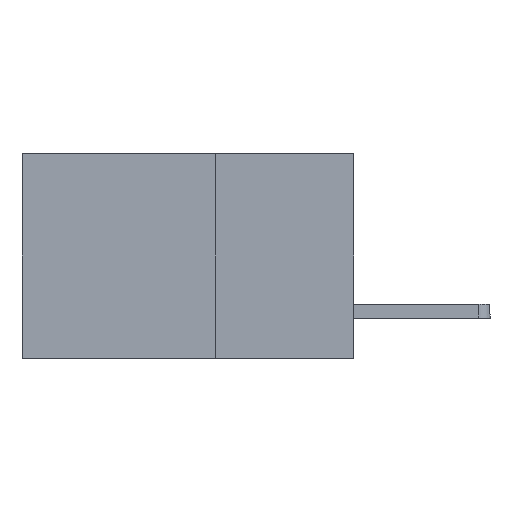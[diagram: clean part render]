
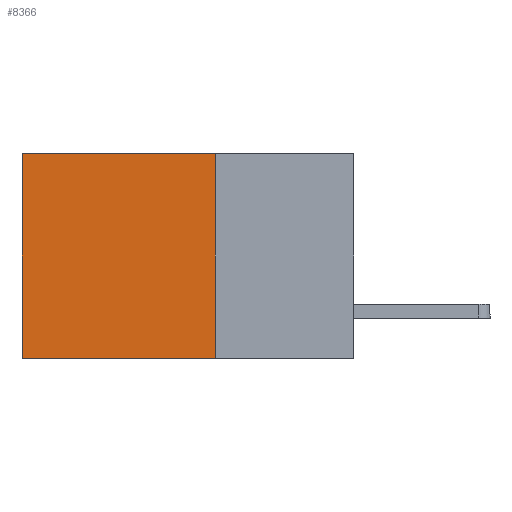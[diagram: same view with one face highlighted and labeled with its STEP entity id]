
A CAD part, left-side view. The second image highlights one B-rep face of the part: STEP entity #8366.
In plain terms, the highlighted planar face has unit normal (-1, 0, 0).
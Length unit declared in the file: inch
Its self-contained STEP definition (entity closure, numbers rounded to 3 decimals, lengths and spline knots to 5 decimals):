
#28 = LINE ( 'NONE', #761, #9189 ) ;
#244 = VECTOR ( 'NONE', #1741, 39.37008 ) ;
#370 = DIRECTION ( 'NONE',  ( 0., 1., 0. ) ) ;
#462 = ORIENTED_EDGE ( 'NONE', *, *, #7740, .T. ) ;
#761 = CARTESIAN_POINT ( 'NONE',  ( 0.2875, 0.6, 0. ) ) ;
#771 = CARTESIAN_POINT ( 'NONE',  ( 0.2875, 0.25, -0.37 ) ) ;
#1051 = VERTEX_POINT ( 'NONE', #2769 ) ;
#1451 = EDGE_LOOP ( 'NONE', ( #462, #9881, #8001, #5736 ) ) ;
#1741 = DIRECTION ( 'NONE',  ( 0., 1., 0. ) ) ;
#1756 = DIRECTION ( 'NONE',  ( 1., 0., 0. ) ) ;
#1991 = LINE ( 'NONE', #7699, #8394 ) ;
#2594 = EDGE_CURVE ( 'NONE', #10038, #2870, #1991, .T. ) ;
#2769 = CARTESIAN_POINT ( 'NONE',  ( 0.2875, 0.6, -0.37 ) ) ;
#2828 = LINE ( 'NONE', #771, #244 ) ;
#2870 = VERTEX_POINT ( 'NONE', #9667 ) ;
#4495 = PLANE ( 'NONE',  #5486 ) ;
#4669 = VERTEX_POINT ( 'NONE', #6980 ) ;
#4952 = EDGE_CURVE ( 'NONE', #2870, #1051, #2828, .T. ) ;
#4968 = LINE ( 'NONE', #9167, #5514 ) ;
#5260 = FACE_OUTER_BOUND ( 'NONE', #1451, .T. ) ;
#5486 = AXIS2_PLACEMENT_3D ( 'NONE', #7082, #1756, #7900 ) ;
#5514 = VECTOR ( 'NONE', #370, 39.37008 ) ;
#5736 = ORIENTED_EDGE ( 'NONE', *, *, #8901, .T. ) ;
#6980 = CARTESIAN_POINT ( 'NONE',  ( 0.2875, 0.6, 0. ) ) ;
#7082 = CARTESIAN_POINT ( 'NONE',  ( 0.2875, 0.25, 0. ) ) ;
#7569 = DIRECTION ( 'NONE',  ( 0., 0., -1. ) ) ;
#7699 = CARTESIAN_POINT ( 'NONE',  ( 0.2875, 0.25, 0. ) ) ;
#7740 = EDGE_CURVE ( 'NONE', #4669, #1051, #28, .T. ) ;
#7900 = DIRECTION ( 'NONE',  ( 0., 0., -1. ) ) ;
#8001 = ORIENTED_EDGE ( 'NONE', *, *, #2594, .F. ) ;
#8366 = ADVANCED_FACE ( 'NONE', ( #5260 ), #4495, .F. ) ;
#8394 = VECTOR ( 'NONE', #7569, 39.37008 ) ;
#8901 = EDGE_CURVE ( 'NONE', #10038, #4669, #4968, .T. ) ;
#9167 = CARTESIAN_POINT ( 'NONE',  ( 0.2875, 0.25, 0. ) ) ;
#9189 = VECTOR ( 'NONE', #11030, 39.37008 ) ;
#9667 = CARTESIAN_POINT ( 'NONE',  ( 0.2875, 0.25, -0.37 ) ) ;
#9881 = ORIENTED_EDGE ( 'NONE', *, *, #4952, .F. ) ;
#10038 = VERTEX_POINT ( 'NONE', #10405 ) ;
#10405 = CARTESIAN_POINT ( 'NONE',  ( 0.2875, 0.25, 0. ) ) ;
#11030 = DIRECTION ( 'NONE',  ( 0., 0., -1. ) ) ;
